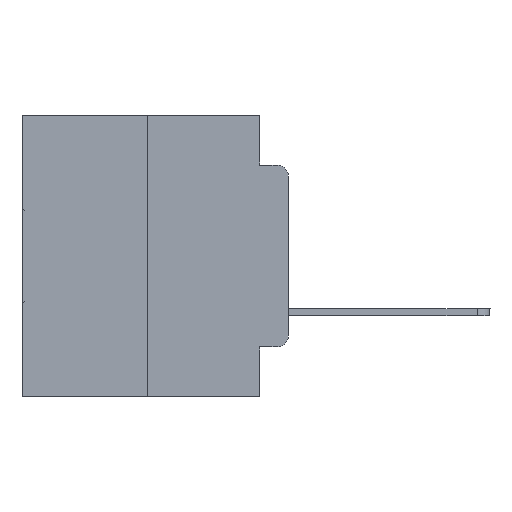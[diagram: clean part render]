
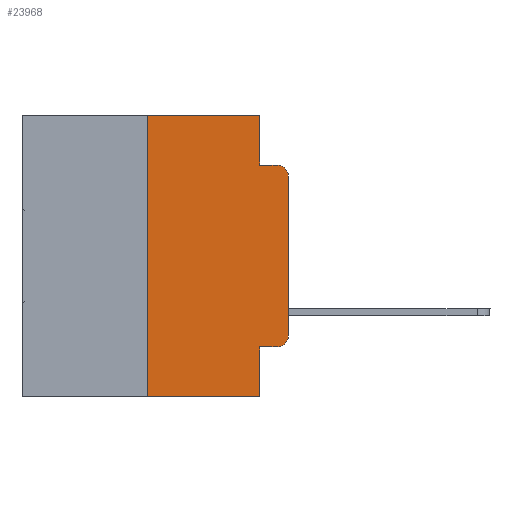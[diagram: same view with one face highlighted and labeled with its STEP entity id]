
A CAD part, left-side view. The second image highlights one B-rep face of the part: STEP entity #23968.
In plain terms, the highlighted planar face has unit normal (-1, 0, 0).
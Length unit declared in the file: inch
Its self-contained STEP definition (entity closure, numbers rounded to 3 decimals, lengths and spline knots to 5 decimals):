
#359 = CARTESIAN_POINT ( 'NONE',  ( 0., 0.25, -0.5 ) ) ;
#530 = CARTESIAN_POINT ( 'NONE',  ( 0., 0.02, -0.4115 ) ) ;
#724 = LINE ( 'NONE', #22082, #8531 ) ;
#787 = LINE ( 'NONE', #7361, #22340 ) ;
#1650 = DIRECTION ( 'NONE',  ( 0., 0., -1. ) ) ;
#1768 = ORIENTED_EDGE ( 'NONE', *, *, #29304, .T. ) ;
#3114 = CARTESIAN_POINT ( 'NONE',  ( 0., 0.051, -0.4115 ) ) ;
#3410 = DIRECTION ( 'NONE',  ( 0., 0., 1. ) ) ;
#3926 = PLANE ( 'NONE',  #14848 ) ;
#4124 = ORIENTED_EDGE ( 'NONE', *, *, #9489, .F. ) ;
#4190 = EDGE_CURVE ( 'NONE', #24772, #26481, #30046, .T. ) ;
#4446 = VECTOR ( 'NONE', #5550, 39.37008 ) ;
#4506 = DIRECTION ( 'NONE',  ( 0., 0., -1. ) ) ;
#5098 = DIRECTION ( 'NONE',  ( 0., 0., -1. ) ) ;
#5550 = DIRECTION ( 'NONE',  ( 0., 0., 1. ) ) ;
#5958 = DIRECTION ( 'NONE',  ( 0., -1., 0. ) ) ;
#6521 = VERTEX_POINT ( 'NONE', #21104 ) ;
#6539 = VECTOR ( 'NONE', #12252, 39.37008 ) ;
#6721 = CARTESIAN_POINT ( 'NONE',  ( 0., 0.02, -0.0885 ) ) ;
#6809 = VECTOR ( 'NONE', #24135, 39.37008 ) ;
#6881 = DIRECTION ( 'NONE',  ( -1., 0., 0. ) ) ;
#7361 = CARTESIAN_POINT ( 'NONE',  ( 0., 0.051, 0. ) ) ;
#7696 = CARTESIAN_POINT ( 'NONE',  ( 0., 0.051, 0. ) ) ;
#8392 = CARTESIAN_POINT ( 'NONE',  ( 0., 0.02, -0.3915 ) ) ;
#8531 = VECTOR ( 'NONE', #26784, 39.37008 ) ;
#8742 = CARTESIAN_POINT ( 'NONE',  ( 0., 0.25, 0. ) ) ;
#8818 = DIRECTION ( 'NONE',  ( 0., 0., -1. ) ) ;
#8977 = ORIENTED_EDGE ( 'NONE', *, *, #21530, .T. ) ;
#9489 = EDGE_CURVE ( 'NONE', #20780, #25658, #787, .T. ) ;
#10547 = VECTOR ( 'NONE', #21383, 39.37008 ) ;
#10761 = VERTEX_POINT ( 'NONE', #23369 ) ;
#10768 = VERTEX_POINT ( 'NONE', #6721 ) ;
#10987 = EDGE_CURVE ( 'NONE', #14028, #20780, #25058, .T. ) ;
#11031 = EDGE_CURVE ( 'NONE', #6521, #26481, #18697, .T. ) ;
#12049 = VECTOR ( 'NONE', #3410, 39.37008 ) ;
#12252 = DIRECTION ( 'NONE',  ( 0., -1., 0. ) ) ;
#13372 = AXIS2_PLACEMENT_3D ( 'NONE', #25717, #6881, #4506 ) ;
#13719 = EDGE_LOOP ( 'NONE', ( #22498, #1768, #27997, #4124, #20683, #17297, #14891, #15413, #30205, #8977 ) ) ;
#13898 = LINE ( 'NONE', #24629, #12049 ) ;
#14028 = VERTEX_POINT ( 'NONE', #8742 ) ;
#14303 = CARTESIAN_POINT ( 'NONE',  ( 0., 0.051, 0. ) ) ;
#14384 = VECTOR ( 'NONE', #5958, 39.37008 ) ;
#14848 = AXIS2_PLACEMENT_3D ( 'NONE', #22955, #27756, #1650 ) ;
#14891 = ORIENTED_EDGE ( 'NONE', *, *, #4190, .T. ) ;
#15017 = EDGE_CURVE ( 'NONE', #6521, #16382, #19184, .T. ) ;
#15333 = CARTESIAN_POINT ( 'NONE',  ( 0., 0.051, -0.0885 ) ) ;
#15413 = ORIENTED_EDGE ( 'NONE', *, *, #11031, .F. ) ;
#16382 = VERTEX_POINT ( 'NONE', #530 ) ;
#17297 = ORIENTED_EDGE ( 'NONE', *, *, #30816, .F. ) ;
#18084 = FACE_OUTER_BOUND ( 'NONE', #13719, .T. ) ;
#18369 = EDGE_CURVE ( 'NONE', #25658, #10768, #724, .T. ) ;
#18697 = LINE ( 'NONE', #14303, #6809 ) ;
#19184 = LINE ( 'NONE', #3114, #6539 ) ;
#19236 = CARTESIAN_POINT ( 'NONE',  ( 0., 0.051, -0.5 ) ) ;
#19598 = CARTESIAN_POINT ( 'NONE',  ( 0., 0., -0.3915 ) ) ;
#19610 = AXIS2_PLACEMENT_3D ( 'NONE', #8392, #25143, #8818 ) ;
#20406 = LINE ( 'NONE', #26467, #4446 ) ;
#20683 = ORIENTED_EDGE ( 'NONE', *, *, #10987, .F. ) ;
#20780 = VERTEX_POINT ( 'NONE', #7696 ) ;
#21104 = CARTESIAN_POINT ( 'NONE',  ( 0., 0.051, -0.4115 ) ) ;
#21383 = DIRECTION ( 'NONE',  ( 0., -1., 0. ) ) ;
#21521 = EDGE_CURVE ( 'NONE', #30116, #10761, #13898, .T. ) ;
#21530 = EDGE_CURVE ( 'NONE', #16382, #30116, #23596, .T. ) ;
#22082 = CARTESIAN_POINT ( 'NONE',  ( 0., 0.051, -0.0885 ) ) ;
#22340 = VECTOR ( 'NONE', #5098, 39.37008 ) ;
#22498 = ORIENTED_EDGE ( 'NONE', *, *, #21521, .T. ) ;
#22955 = CARTESIAN_POINT ( 'NONE',  ( 0., 0.473, 0. ) ) ;
#23369 = CARTESIAN_POINT ( 'NONE',  ( 0., 0., -0.1085 ) ) ;
#23596 = CIRCLE ( 'NONE', #19610, 0.02 ) ;
#23968 = ADVANCED_FACE ( 'NONE', ( #18084 ), #3926, .F. ) ;
#24135 = DIRECTION ( 'NONE',  ( 0., 0., -1. ) ) ;
#24629 = CARTESIAN_POINT ( 'NONE',  ( 0., 0., 0. ) ) ;
#24772 = VERTEX_POINT ( 'NONE', #359 ) ;
#24892 = CARTESIAN_POINT ( 'NONE',  ( 0., 0.473, -0.5 ) ) ;
#25058 = LINE ( 'NONE', #28496, #10547 ) ;
#25143 = DIRECTION ( 'NONE',  ( -1., 0., 0. ) ) ;
#25658 = VERTEX_POINT ( 'NONE', #15333 ) ;
#25717 = CARTESIAN_POINT ( 'NONE',  ( 0., 0.02, -0.1085 ) ) ;
#26467 = CARTESIAN_POINT ( 'NONE',  ( 0., 0.25, 0. ) ) ;
#26481 = VERTEX_POINT ( 'NONE', #19236 ) ;
#26784 = DIRECTION ( 'NONE',  ( 0., -1., 0. ) ) ;
#26881 = CIRCLE ( 'NONE', #13372, 0.02 ) ;
#27756 = DIRECTION ( 'NONE',  ( 1., 0., 0. ) ) ;
#27997 = ORIENTED_EDGE ( 'NONE', *, *, #18369, .F. ) ;
#28496 = CARTESIAN_POINT ( 'NONE',  ( 0., 0.473, 0. ) ) ;
#29304 = EDGE_CURVE ( 'NONE', #10761, #10768, #26881, .T. ) ;
#30046 = LINE ( 'NONE', #24892, #14384 ) ;
#30116 = VERTEX_POINT ( 'NONE', #19598 ) ;
#30205 = ORIENTED_EDGE ( 'NONE', *, *, #15017, .T. ) ;
#30816 = EDGE_CURVE ( 'NONE', #24772, #14028, #20406, .T. ) ;
